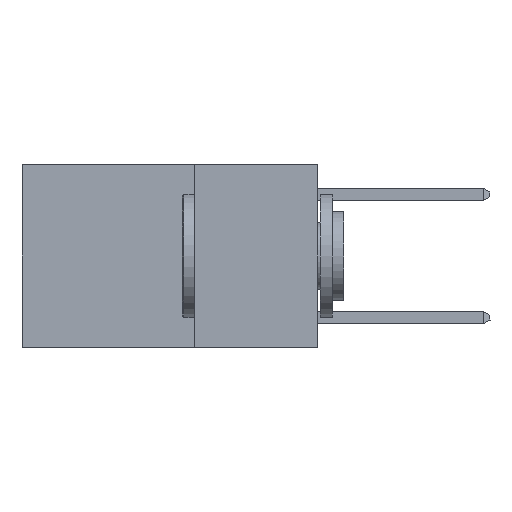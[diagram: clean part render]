
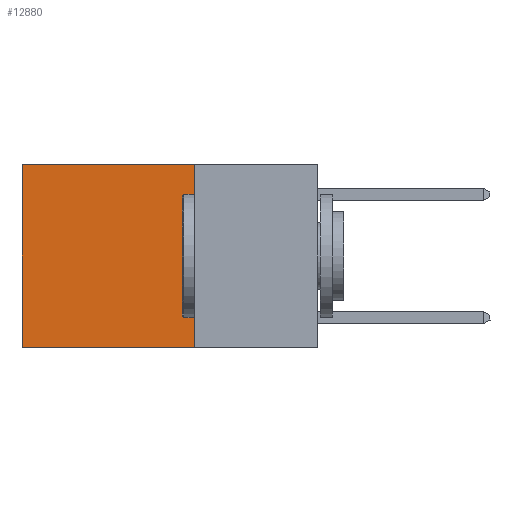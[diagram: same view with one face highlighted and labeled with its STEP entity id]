
A CAD part, left-side view. The second image highlights one B-rep face of the part: STEP entity #12880.
In plain terms, the highlighted planar face has unit normal (-1, 0, 0).
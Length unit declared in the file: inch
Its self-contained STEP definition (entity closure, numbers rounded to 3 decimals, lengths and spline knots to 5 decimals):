
#170 = DIRECTION ( 'NONE',  ( 0., 0., -1. ) ) ;
#206 = EDGE_CURVE ( 'NONE', #12805, #11993, #8491, .T. ) ;
#984 = CARTESIAN_POINT ( 'NONE',  ( 0.2625, 0.25, 0. ) ) ;
#1269 = EDGE_LOOP ( 'NONE', ( #2057, #8080, #10784, #4371 ) ) ;
#2057 = ORIENTED_EDGE ( 'NONE', *, *, #5966, .T. ) ;
#2133 = CARTESIAN_POINT ( 'NONE',  ( 0.2625, 0.25, 0. ) ) ;
#2362 = VERTEX_POINT ( 'NONE', #2686 ) ;
#2686 = CARTESIAN_POINT ( 'NONE',  ( 0.2625, 0.6, 0. ) ) ;
#2891 = VECTOR ( 'NONE', #13330, 39.37008 ) ;
#3317 = DIRECTION ( 'NONE',  ( 0., 0., -1. ) ) ;
#3527 = CARTESIAN_POINT ( 'NONE',  ( 0.2625, 0.25, 0. ) ) ;
#4211 = CARTESIAN_POINT ( 'NONE',  ( 0.2625, 0.25, -0.37 ) ) ;
#4371 = ORIENTED_EDGE ( 'NONE', *, *, #10054, .T. ) ;
#4630 = DIRECTION ( 'NONE',  ( 0., 0., -1. ) ) ;
#4988 = VECTOR ( 'NONE', #3317, 39.37008 ) ;
#5338 = LINE ( 'NONE', #13509, #4988 ) ;
#5966 = EDGE_CURVE ( 'NONE', #2362, #11993, #5338, .T. ) ;
#6123 = VECTOR ( 'NONE', #170, 39.37008 ) ;
#6153 = EDGE_CURVE ( 'NONE', #6966, #12805, #11533, .T. ) ;
#6966 = VERTEX_POINT ( 'NONE', #984 ) ;
#7110 = AXIS2_PLACEMENT_3D ( 'NONE', #3527, #10755, #4630 ) ;
#7482 = DIRECTION ( 'NONE',  ( 0., 1., 0. ) ) ;
#7613 = CARTESIAN_POINT ( 'NONE',  ( 0.2625, 0.25, -0.37 ) ) ;
#8080 = ORIENTED_EDGE ( 'NONE', *, *, #206, .F. ) ;
#8491 = LINE ( 'NONE', #4211, #2891 ) ;
#9729 = PLANE ( 'NONE',  #7110 ) ;
#10054 = EDGE_CURVE ( 'NONE', #6966, #2362, #12071, .T. ) ;
#10755 = DIRECTION ( 'NONE',  ( 1., 0., 0. ) ) ;
#10780 = CARTESIAN_POINT ( 'NONE',  ( 0.2625, 0.25, 0. ) ) ;
#10784 = ORIENTED_EDGE ( 'NONE', *, *, #6153, .F. ) ;
#11533 = LINE ( 'NONE', #10780, #6123 ) ;
#11766 = VECTOR ( 'NONE', #7482, 39.37008 ) ;
#11993 = VERTEX_POINT ( 'NONE', #12273 ) ;
#12071 = LINE ( 'NONE', #2133, #11766 ) ;
#12273 = CARTESIAN_POINT ( 'NONE',  ( 0.2625, 0.6, -0.37 ) ) ;
#12805 = VERTEX_POINT ( 'NONE', #7613 ) ;
#12880 = ADVANCED_FACE ( 'NONE', ( #13326 ), #9729, .F. ) ;
#13326 = FACE_OUTER_BOUND ( 'NONE', #1269, .T. ) ;
#13330 = DIRECTION ( 'NONE',  ( 0., 1., 0. ) ) ;
#13509 = CARTESIAN_POINT ( 'NONE',  ( 0.2625, 0.6, 0. ) ) ;
